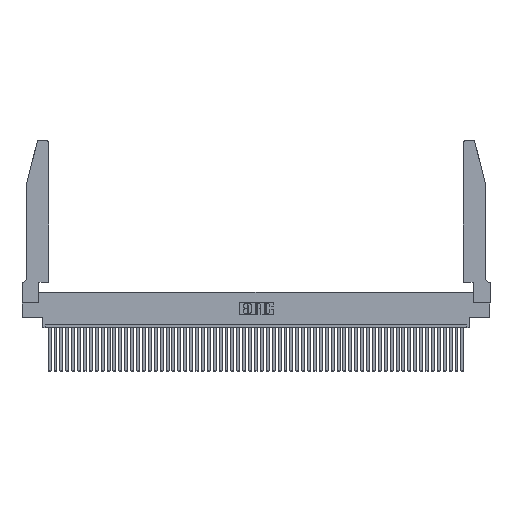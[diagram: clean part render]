
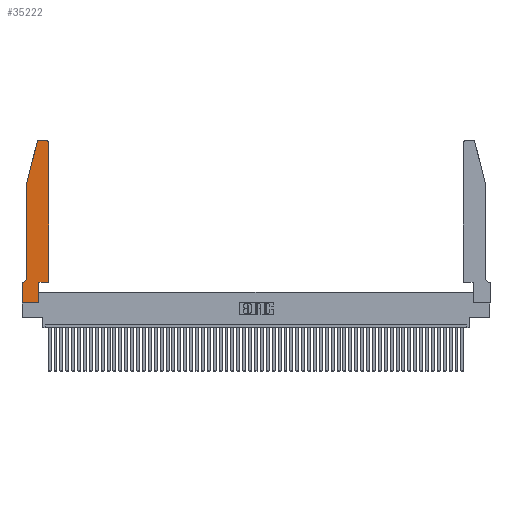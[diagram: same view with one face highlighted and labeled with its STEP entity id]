
A CAD part, top view. The second image highlights one B-rep face of the part: STEP entity #35222.
In plain terms, the highlighted planar face has unit normal (0, 0, 1).
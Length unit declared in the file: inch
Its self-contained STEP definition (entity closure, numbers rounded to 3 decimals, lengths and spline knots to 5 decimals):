
#400 = DIRECTION ( 'NONE',  ( -1., 0., 0. ) ) ;
#923 = AXIS2_PLACEMENT_3D ( 'NONE', #36004, #10764, #1925 ) ;
#1925 = DIRECTION ( 'NONE',  ( 1., 0., 0. ) ) ;
#2466 = VECTOR ( 'NONE', #25197, 39.37008 ) ;
#2760 = CARTESIAN_POINT ( 'NONE',  ( 0.25487, 2.72718, 0.37 ) ) ;
#3258 = AXIS2_PLACEMENT_3D ( 'NONE', #27938, #53033, #3429 ) ;
#3345 = ORIENTED_EDGE ( 'NONE', *, *, #5610, .T. ) ;
#3429 = DIRECTION ( 'NONE',  ( 1., 0., 0. ) ) ;
#3802 = ORIENTED_EDGE ( 'NONE', *, *, #35648, .T. ) ;
#3825 = CARTESIAN_POINT ( 'NONE',  ( 0.4205, 2.75, 0.37 ) ) ;
#4456 = ORIENTED_EDGE ( 'NONE', *, *, #32266, .T. ) ;
#4505 = EDGE_CURVE ( 'NONE', #32148, #6131, #47072, .T. ) ;
#4659 = DIRECTION ( 'NONE',  ( 0., 0., -1. ) ) ;
#4773 = CARTESIAN_POINT ( 'NONE',  ( 0.4505, 0.35, 0.37 ) ) ;
#5171 = CARTESIAN_POINT ( 'NONE',  ( 0., 0.35, 0.37 ) ) ;
#5198 = ORIENTED_EDGE ( 'NONE', *, *, #25468, .T. ) ;
#5610 = EDGE_CURVE ( 'NONE', #22107, #32148, #17674, .T. ) ;
#5883 = VERTEX_POINT ( 'NONE', #9426 ) ;
#6131 = VERTEX_POINT ( 'NONE', #15621 ) ;
#6239 = VECTOR ( 'NONE', #38490, 39.37008 ) ;
#6534 = CARTESIAN_POINT ( 'NONE',  ( 0.0755, 2., 0.37 ) ) ;
#6779 = ORIENTED_EDGE ( 'NONE', *, *, #51495, .T. ) ;
#7802 = DIRECTION ( 'NONE',  ( 0., -1., 0. ) ) ;
#8622 = CIRCLE ( 'NONE', #52784, 0.07 ) ;
#8646 = ORIENTED_EDGE ( 'NONE', *, *, #32681, .T. ) ;
#8783 = ORIENTED_EDGE ( 'NONE', *, *, #30654, .T. ) ;
#9140 = VECTOR ( 'NONE', #10371, 39.37008 ) ;
#9426 = CARTESIAN_POINT ( 'NONE',  ( 0.0055, 0.35, 0.37 ) ) ;
#10371 = DIRECTION ( 'NONE',  ( 1., 0., 0. ) ) ;
#10451 = ORIENTED_EDGE ( 'NONE', *, *, #25034, .T. ) ;
#10529 = DIRECTION ( 'NONE',  ( 0., -1., 0. ) ) ;
#10764 = DIRECTION ( 'NONE',  ( 0., 0., 1. ) ) ;
#11216 = CARTESIAN_POINT ( 'NONE',  ( 0., 0.35, 0.37 ) ) ;
#11956 = EDGE_LOOP ( 'NONE', ( #3802, #6779, #8783, #20327, #8646, #53244, #3345, #32960, #10451, #53052, #4456, #5198 ) ) ;
#12008 = VERTEX_POINT ( 'NONE', #4773 ) ;
#12064 = CARTESIAN_POINT ( 'NONE',  ( 0.0755, 2., 0.37 ) ) ;
#13242 = DIRECTION ( 'NONE',  ( 0., 1., 0. ) ) ;
#13342 = EDGE_CURVE ( 'NONE', #35456, #52544, #53482, .T. ) ;
#14375 = VECTOR ( 'NONE', #7802, 39.37008 ) ;
#14530 = LINE ( 'NONE', #38791, #52457 ) ;
#14717 = VERTEX_POINT ( 'NONE', #47989 ) ;
#15621 = CARTESIAN_POINT ( 'NONE',  ( 0.2865, 0., 0.37 ) ) ;
#16190 = CIRCLE ( 'NONE', #923, 0.03 ) ;
#16786 = CARTESIAN_POINT ( 'NONE',  ( 0.284, 2.75, 0.37 ) ) ;
#17674 = LINE ( 'NONE', #24285, #14375 ) ;
#20018 = PLANE ( 'NONE',  #44441 ) ;
#20222 = DIRECTION ( 'NONE',  ( 1., 0., 0. ) ) ;
#20327 = ORIENTED_EDGE ( 'NONE', *, *, #13342, .T. ) ;
#21506 = CIRCLE ( 'NONE', #3258, 0.03 ) ;
#21602 = LINE ( 'NONE', #26832, #9140 ) ;
#22107 = VERTEX_POINT ( 'NONE', #5171 ) ;
#22852 = VECTOR ( 'NONE', #20222, 39.37008 ) ;
#24285 = CARTESIAN_POINT ( 'NONE',  ( 0., 0., 0.37 ) ) ;
#24396 = CARTESIAN_POINT ( 'NONE',  ( 0.2865, 0.35, 0.37 ) ) ;
#25034 = EDGE_CURVE ( 'NONE', #6131, #14717, #32654, .T. ) ;
#25197 = DIRECTION ( 'NONE',  ( 0., 1., 0. ) ) ;
#25468 = EDGE_CURVE ( 'NONE', #26573, #28606, #16190, .T. ) ;
#25651 = DIRECTION ( 'NONE',  ( -1., 0., 0. ) ) ;
#26573 = VERTEX_POINT ( 'NONE', #32090 ) ;
#26832 = CARTESIAN_POINT ( 'NONE',  ( 0.4505, 0.35, 0.37 ) ) ;
#27808 = VERTEX_POINT ( 'NONE', #2760 ) ;
#27938 = CARTESIAN_POINT ( 'NONE',  ( 0.284, 2.72, 0.37 ) ) ;
#28594 = FACE_OUTER_BOUND ( 'NONE', #11956, .T. ) ;
#28606 = VERTEX_POINT ( 'NONE', #3825 ) ;
#29013 = LINE ( 'NONE', #30072, #33569 ) ;
#30072 = CARTESIAN_POINT ( 'NONE',  ( 0.4505, 0.35, 0.37 ) ) ;
#30654 = EDGE_CURVE ( 'NONE', #27808, #35456, #37629, .T. ) ;
#32090 = CARTESIAN_POINT ( 'NONE',  ( 0.4505, 2.72, 0.37 ) ) ;
#32148 = VERTEX_POINT ( 'NONE', #43892 ) ;
#32266 = EDGE_CURVE ( 'NONE', #12008, #26573, #29013, .T. ) ;
#32496 = VECTOR ( 'NONE', #10529, 39.37008 ) ;
#32654 = LINE ( 'NONE', #24396, #2466 ) ;
#32681 = EDGE_CURVE ( 'NONE', #52544, #5883, #8622, .T. ) ;
#32960 = ORIENTED_EDGE ( 'NONE', *, *, #4505, .T. ) ;
#33569 = VECTOR ( 'NONE', #13242, 39.37008 ) ;
#35222 = ADVANCED_FACE ( 'NONE', ( #28594 ), #20018, .T. ) ;
#35456 = VERTEX_POINT ( 'NONE', #12064 ) ;
#35648 = EDGE_CURVE ( 'NONE', #28606, #39884, #42278, .T. ) ;
#36004 = CARTESIAN_POINT ( 'NONE',  ( 0.4205, 2.72, 0.37 ) ) ;
#37629 = LINE ( 'NONE', #50601, #6239 ) ;
#38261 = CARTESIAN_POINT ( 'NONE',  ( 0.0055, 0.42, 0.37 ) ) ;
#38490 = DIRECTION ( 'NONE',  ( -0.239, -0.971, 0. ) ) ;
#38791 = CARTESIAN_POINT ( 'NONE',  ( 0.0755, 0.35, 0.37 ) ) ;
#39884 = VERTEX_POINT ( 'NONE', #16786 ) ;
#40500 = DIRECTION ( 'NONE',  ( 0., 0., 1. ) ) ;
#40686 = DIRECTION ( 'NONE',  ( 1., 0., 0. ) ) ;
#41208 = EDGE_CURVE ( 'NONE', #5883, #22107, #14530, .T. ) ;
#42278 = LINE ( 'NONE', #52055, #48849 ) ;
#42609 = CARTESIAN_POINT ( 'NONE',  ( 0.0755, 0.42, 0.37 ) ) ;
#43892 = CARTESIAN_POINT ( 'NONE',  ( 0., 0., 0.37 ) ) ;
#44342 = DIRECTION ( 'NONE',  ( -1., 0., 0. ) ) ;
#44438 = EDGE_CURVE ( 'NONE', #14717, #12008, #21602, .T. ) ;
#44441 = AXIS2_PLACEMENT_3D ( 'NONE', #11216, #40500, #40686 ) ;
#45623 = CARTESIAN_POINT ( 'NONE',  ( 0., 0., 0.37 ) ) ;
#47072 = LINE ( 'NONE', #45623, #22852 ) ;
#47989 = CARTESIAN_POINT ( 'NONE',  ( 0.2865, 0.35, 0.37 ) ) ;
#48849 = VECTOR ( 'NONE', #44342, 39.37008 ) ;
#50601 = CARTESIAN_POINT ( 'NONE',  ( 0.0755, 2., 0.37 ) ) ;
#51495 = EDGE_CURVE ( 'NONE', #39884, #27808, #21506, .T. ) ;
#52055 = CARTESIAN_POINT ( 'NONE',  ( 0.2605, 2.75, 0.37 ) ) ;
#52457 = VECTOR ( 'NONE', #400, 39.37008 ) ;
#52544 = VERTEX_POINT ( 'NONE', #42609 ) ;
#52784 = AXIS2_PLACEMENT_3D ( 'NONE', #38261, #4659, #25651 ) ;
#53033 = DIRECTION ( 'NONE',  ( 0., 0., 1. ) ) ;
#53052 = ORIENTED_EDGE ( 'NONE', *, *, #44438, .T. ) ;
#53244 = ORIENTED_EDGE ( 'NONE', *, *, #41208, .T. ) ;
#53482 = LINE ( 'NONE', #6534, #32496 ) ;
